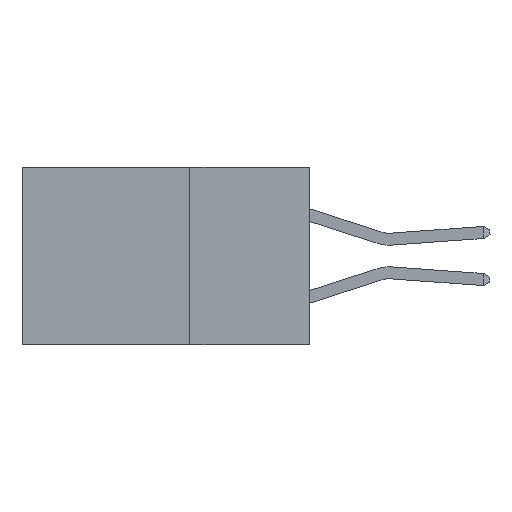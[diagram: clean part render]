
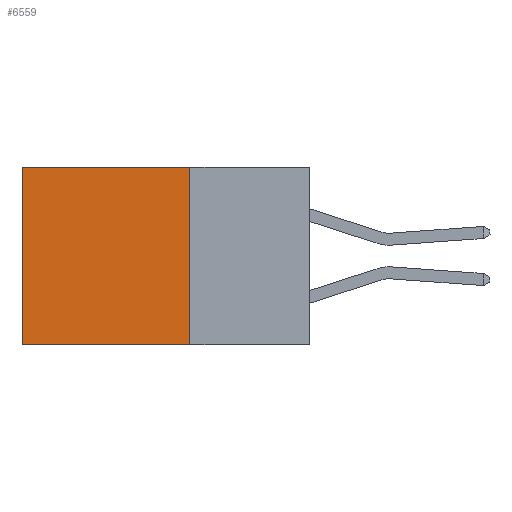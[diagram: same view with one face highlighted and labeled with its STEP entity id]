
A CAD part, left-side view. The second image highlights one B-rep face of the part: STEP entity #6559.
In plain terms, the highlighted planar face has unit normal (-1, 0, 0).
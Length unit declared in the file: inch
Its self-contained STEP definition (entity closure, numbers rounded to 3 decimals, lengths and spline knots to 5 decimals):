
#286 = DIRECTION ( 'NONE',  ( 0., 0., -1. ) ) ;
#303 = VECTOR ( 'NONE', #6574, 39.37008 ) ;
#521 = ORIENTED_EDGE ( 'NONE', *, *, #6841, .F. ) ;
#684 = ORIENTED_EDGE ( 'NONE', *, *, #9711, .T. ) ;
#770 = CARTESIAN_POINT ( 'NONE',  ( 0.298, 0.25, 0. ) ) ;
#882 = ORIENTED_EDGE ( 'NONE', *, *, #5929, .F. ) ;
#1108 = EDGE_LOOP ( 'NONE', ( #6749, #882, #521, #684 ) ) ;
#1546 = AXIS2_PLACEMENT_3D ( 'NONE', #770, #6563, #1637 ) ;
#1637 = DIRECTION ( 'NONE',  ( 0., 0., -1. ) ) ;
#1638 = VECTOR ( 'NONE', #286, 39.37008 ) ;
#2179 = EDGE_CURVE ( 'NONE', #6762, #9263, #6329, .T. ) ;
#2311 = FACE_OUTER_BOUND ( 'NONE', #1108, .T. ) ;
#2811 = LINE ( 'NONE', #5768, #303 ) ;
#2834 = CARTESIAN_POINT ( 'NONE',  ( 0.298, 0.25, 0. ) ) ;
#3892 = VECTOR ( 'NONE', #9228, 39.37008 ) ;
#4456 = CARTESIAN_POINT ( 'NONE',  ( 0.298, 0.25, 0. ) ) ;
#4929 = PLANE ( 'NONE',  #1546 ) ;
#5224 = VERTEX_POINT ( 'NONE', #9434 ) ;
#5741 = VECTOR ( 'NONE', #7137, 39.37008 ) ;
#5768 = CARTESIAN_POINT ( 'NONE',  ( 0.298, 0.25, -0.37 ) ) ;
#5929 = EDGE_CURVE ( 'NONE', #9928, #9263, #2811, .T. ) ;
#6329 = LINE ( 'NONE', #8365, #3892 ) ;
#6559 = ADVANCED_FACE ( 'NONE', ( #2311 ), #4929, .F. ) ;
#6563 = DIRECTION ( 'NONE',  ( 1., 0., 0. ) ) ;
#6574 = DIRECTION ( 'NONE',  ( 0., 1., 0. ) ) ;
#6749 = ORIENTED_EDGE ( 'NONE', *, *, #2179, .T. ) ;
#6762 = VERTEX_POINT ( 'NONE', #9148 ) ;
#6841 = EDGE_CURVE ( 'NONE', #5224, #9928, #8151, .T. ) ;
#7137 = DIRECTION ( 'NONE',  ( 0., 1., 0. ) ) ;
#7504 = CARTESIAN_POINT ( 'NONE',  ( 0.298, 0.25, -0.37 ) ) ;
#7862 = LINE ( 'NONE', #2834, #5741 ) ;
#8151 = LINE ( 'NONE', #4456, #1638 ) ;
#8365 = CARTESIAN_POINT ( 'NONE',  ( 0.298, 0.6, 0. ) ) ;
#9148 = CARTESIAN_POINT ( 'NONE',  ( 0.298, 0.6, 0. ) ) ;
#9228 = DIRECTION ( 'NONE',  ( 0., 0., -1. ) ) ;
#9263 = VERTEX_POINT ( 'NONE', #10453 ) ;
#9434 = CARTESIAN_POINT ( 'NONE',  ( 0.298, 0.25, 0. ) ) ;
#9711 = EDGE_CURVE ( 'NONE', #5224, #6762, #7862, .T. ) ;
#9928 = VERTEX_POINT ( 'NONE', #7504 ) ;
#10453 = CARTESIAN_POINT ( 'NONE',  ( 0.298, 0.6, -0.37 ) ) ;
